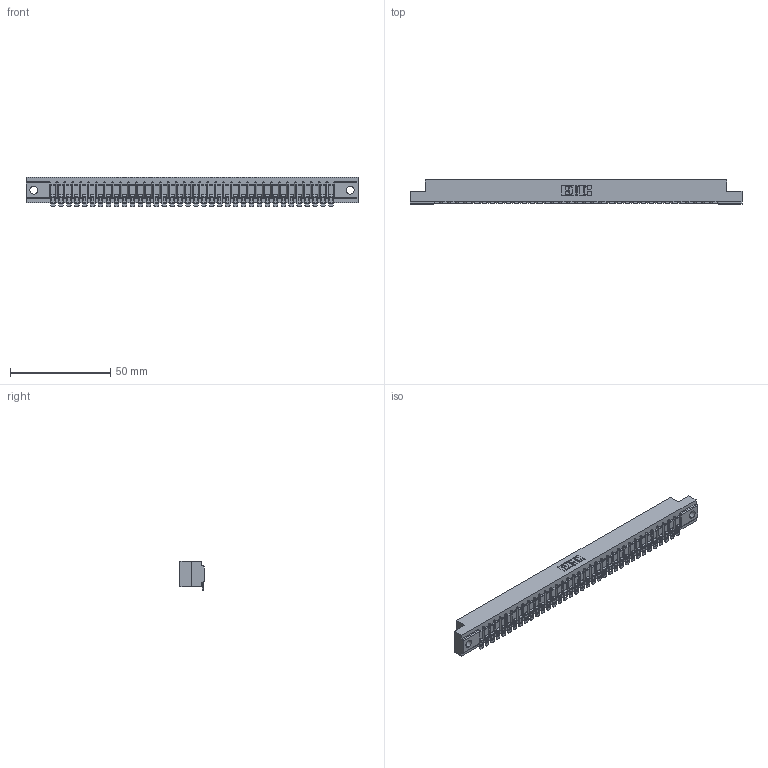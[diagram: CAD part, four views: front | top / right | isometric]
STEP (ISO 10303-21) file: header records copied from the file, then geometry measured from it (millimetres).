
FILE_DESCRIPTION (( 'STEP AP203' ), '1' );
FILE_NAME ('307-036-554-104.STEP', '2019-09-05T08:00:38', ( '' ), ( '' ), 'SwSTEP 2.0', 'SolidWorks 2016', '' );
FILE_SCHEMA (( 'CONFIG_CONTROL_DESIGN' ));
Length unit declared in the file: inch
Products named in the file (3): 307-036-554-104; 307 Part_.156 Dia Mounting Holes; 307-290-002_554
Assembly tree (37 placements, depth 2):
  307-036-554-104
    307 Part_.156 Dia Mounting Holes
    307-290-002_554  x36
Bounding box: 165.66 x 12.01 x 14.52 mm (x, y, z)
Volume: 17589.9 mm3; surface area: 21959.9 mm2
Topology: 37 solids, 37 shells, 3085 faces, 9467 edges, 6210 vertices
Faces by surface type: plane 1740, cylinder 1271, sphere 74
Entity records: 32985 total; most frequent: CARTESIAN_POINT 5568, ORIENTED_EDGE 5556, DIRECTION 5410, EDGE_CURVE 2778, VECTOR 2126, LINE 2126, VERTEX_POINT 1800, AXIS2_PLACEMENT_3D 1642
